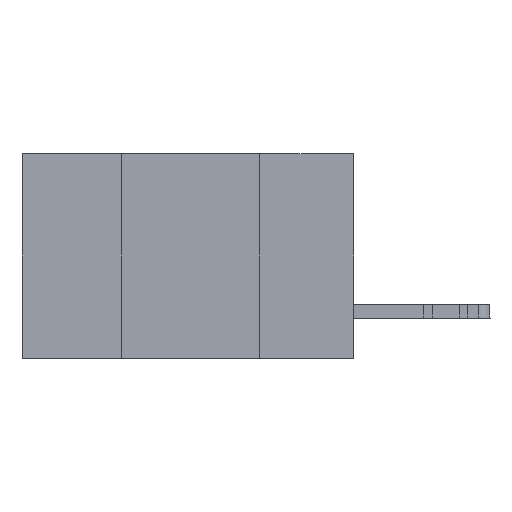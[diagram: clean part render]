
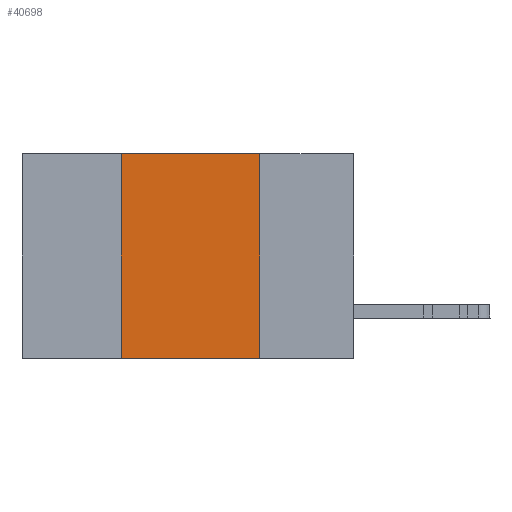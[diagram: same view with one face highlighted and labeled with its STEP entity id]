
A CAD part, left-side view. The second image highlights one B-rep face of the part: STEP entity #40698.
In plain terms, the highlighted planar face has unit normal (-1, 0, 0).
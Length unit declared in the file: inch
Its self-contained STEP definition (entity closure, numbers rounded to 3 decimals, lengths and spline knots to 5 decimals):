
#1813 = EDGE_CURVE ( 'NONE', #28767, #23468, #26587, .T. ) ;
#1872 = VERTEX_POINT ( 'NONE', #32877 ) ;
#2177 = CARTESIAN_POINT ( 'NONE',  ( 0., 0.6, 0. ) ) ;
#2323 = LINE ( 'NONE', #11997, #8439 ) ;
#7452 = CARTESIAN_POINT ( 'NONE',  ( 0., 0.6, -0.37 ) ) ;
#8421 = EDGE_CURVE ( 'NONE', #11319, #23468, #21636, .T. ) ;
#8439 = VECTOR ( 'NONE', #31536, 39.37008 ) ;
#9829 = CARTESIAN_POINT ( 'NONE',  ( 0., 0.42, -0.37 ) ) ;
#10909 = ORIENTED_EDGE ( 'NONE', *, *, #1813, .T. ) ;
#11319 = VERTEX_POINT ( 'NONE', #27080 ) ;
#11997 = CARTESIAN_POINT ( 'NONE',  ( 0., 0.6, 0. ) ) ;
#12340 = LINE ( 'NONE', #25178, #25491 ) ;
#12715 = EDGE_CURVE ( 'NONE', #28767, #1872, #12340, .T. ) ;
#12777 = VECTOR ( 'NONE', #27943, 39.37008 ) ;
#14992 = DIRECTION ( 'NONE',  ( 1., 0., 0. ) ) ;
#15979 = ORIENTED_EDGE ( 'NONE', *, *, #26924, .F. ) ;
#17694 = ORIENTED_EDGE ( 'NONE', *, *, #8421, .F. ) ;
#18152 = PLANE ( 'NONE',  #20424 ) ;
#18358 = DIRECTION ( 'NONE',  ( 0., 0., -1. ) ) ;
#20424 = AXIS2_PLACEMENT_3D ( 'NONE', #2177, #14992, #18358 ) ;
#21636 = LINE ( 'NONE', #31303, #12777 ) ;
#23468 = VERTEX_POINT ( 'NONE', #41111 ) ;
#25178 = CARTESIAN_POINT ( 'NONE',  ( 0., 0.42, 0. ) ) ;
#25491 = VECTOR ( 'NONE', #37987, 39.37008 ) ;
#26587 = LINE ( 'NONE', #7452, #37965 ) ;
#26810 = EDGE_LOOP ( 'NONE', ( #17694, #15979, #33584, #10909 ) ) ;
#26924 = EDGE_CURVE ( 'NONE', #1872, #11319, #2323, .T. ) ;
#27080 = CARTESIAN_POINT ( 'NONE',  ( 0., 0.17, 0. ) ) ;
#27943 = DIRECTION ( 'NONE',  ( 0., 0., -1. ) ) ;
#28767 = VERTEX_POINT ( 'NONE', #9829 ) ;
#31303 = CARTESIAN_POINT ( 'NONE',  ( 0., 0.17, 0. ) ) ;
#31536 = DIRECTION ( 'NONE',  ( 0., -1., 0. ) ) ;
#32877 = CARTESIAN_POINT ( 'NONE',  ( 0., 0.42, 0. ) ) ;
#33292 = DIRECTION ( 'NONE',  ( 0., -1., 0. ) ) ;
#33584 = ORIENTED_EDGE ( 'NONE', *, *, #12715, .F. ) ;
#37274 = FACE_OUTER_BOUND ( 'NONE', #26810, .T. ) ;
#37965 = VECTOR ( 'NONE', #33292, 39.37008 ) ;
#37987 = DIRECTION ( 'NONE',  ( 0., 0., 1. ) ) ;
#40698 = ADVANCED_FACE ( 'NONE', ( #37274 ), #18152, .F. ) ;
#41111 = CARTESIAN_POINT ( 'NONE',  ( 0., 0.17, -0.37 ) ) ;
